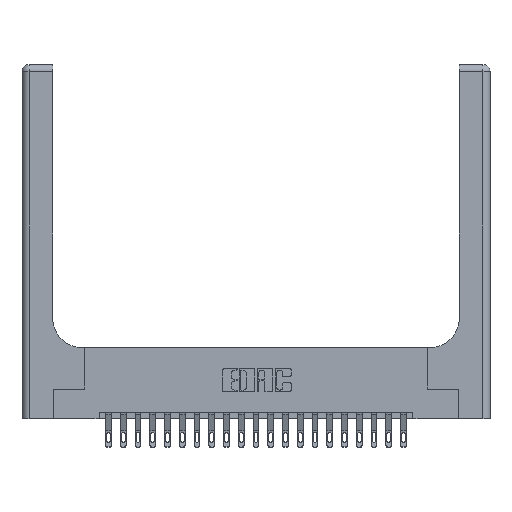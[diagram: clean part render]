
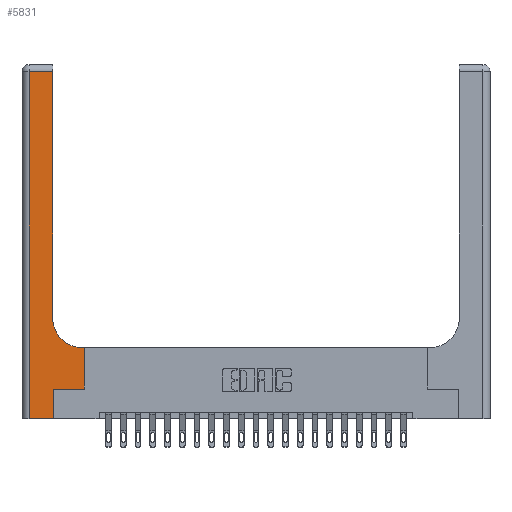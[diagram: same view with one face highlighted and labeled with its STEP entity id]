
A CAD part, top view. The second image highlights one B-rep face of the part: STEP entity #5831.
In plain terms, the highlighted planar face has unit normal (0, 0, 1).
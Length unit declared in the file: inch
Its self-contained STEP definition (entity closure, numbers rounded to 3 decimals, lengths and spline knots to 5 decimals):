
#653 = ORIENTED_EDGE ( 'NONE', *, *, #1979, .T. ) ;
#1203 = EDGE_CURVE ( 'NONE', #4812, #17176, #13345, .T. ) ;
#1388 = CARTESIAN_POINT ( 'NONE',  ( 0.06, 0., 0.37 ) ) ;
#1412 = DIRECTION ( 'NONE',  ( 0., 1., 0. ) ) ;
#1979 = EDGE_CURVE ( 'NONE', #17176, #2848, #15249, .T. ) ;
#2100 = ORIENTED_EDGE ( 'NONE', *, *, #11802, .T. ) ;
#2251 = VECTOR ( 'NONE', #11973, 39.37008 ) ;
#2461 = DIRECTION ( 'NONE',  ( -1., 0., 0. ) ) ;
#2636 = CARTESIAN_POINT ( 'NONE',  ( 0.26, 0.6, 0.37 ) ) ;
#2697 = DIRECTION ( 'NONE',  ( 0., 1., 0. ) ) ;
#2848 = VERTEX_POINT ( 'NONE', #14149 ) ;
#3177 = CARTESIAN_POINT ( 'NONE',  ( 0.51, 0.6, 0.37 ) ) ;
#3280 = ORIENTED_EDGE ( 'NONE', *, *, #10974, .T. ) ;
#3754 = CARTESIAN_POINT ( 'NONE',  ( 0.265, 0., 0.37 ) ) ;
#3916 = CARTESIAN_POINT ( 'NONE',  ( 0., 0., 0.37 ) ) ;
#4311 = ORIENTED_EDGE ( 'NONE', *, *, #11282, .T. ) ;
#4402 = CARTESIAN_POINT ( 'NONE',  ( 0.528, 0.25, 0.37 ) ) ;
#4812 = VERTEX_POINT ( 'NONE', #6133 ) ;
#5831 = ADVANCED_FACE ( 'NONE', ( #19494 ), #12582, .F. ) ;
#6133 = CARTESIAN_POINT ( 'NONE',  ( 0.528, 0.6, 0.37 ) ) ;
#6538 = DIRECTION ( 'NONE',  ( 1., 0., 0. ) ) ;
#6682 = DIRECTION ( 'NONE',  ( 1., 0., 0. ) ) ;
#6958 = VERTEX_POINT ( 'NONE', #17287 ) ;
#7157 = ORIENTED_EDGE ( 'NONE', *, *, #1203, .T. ) ;
#7297 = EDGE_CURVE ( 'NONE', #20458, #9499, #17157, .T. ) ;
#7345 = LINE ( 'NONE', #3916, #10226 ) ;
#7365 = VECTOR ( 'NONE', #1412, 39.37008 ) ;
#7454 = AXIS2_PLACEMENT_3D ( 'NONE', #21672, #19728, #16337 ) ;
#8515 = ORIENTED_EDGE ( 'NONE', *, *, #7297, .T. ) ;
#8756 = VECTOR ( 'NONE', #2697, 39.37008 ) ;
#8896 = CARTESIAN_POINT ( 'NONE',  ( 0.265, 0.25, 0.37 ) ) ;
#9025 = CARTESIAN_POINT ( 'NONE',  ( 0.06, 2.94, 0.37 ) ) ;
#9262 = LINE ( 'NONE', #16222, #17305 ) ;
#9431 = VECTOR ( 'NONE', #6538, 39.37008 ) ;
#9499 = VERTEX_POINT ( 'NONE', #15366 ) ;
#10226 = VECTOR ( 'NONE', #19401, 39.37008 ) ;
#10974 = EDGE_CURVE ( 'NONE', #9499, #4812, #19881, .T. ) ;
#11282 = EDGE_CURVE ( 'NONE', #15295, #21851, #7345, .T. ) ;
#11802 = EDGE_CURVE ( 'NONE', #13769, #15295, #16662, .T. ) ;
#11973 = DIRECTION ( 'NONE',  ( 0., -1., 0. ) ) ;
#12073 = LINE ( 'NONE', #19518, #16566 ) ;
#12582 = PLANE ( 'NONE',  #7454 ) ;
#12653 = EDGE_CURVE ( 'NONE', #21851, #20458, #13720, .T. ) ;
#12925 = DIRECTION ( 'NONE',  ( 0., 1., 0. ) ) ;
#13345 = LINE ( 'NONE', #2636, #22180 ) ;
#13720 = LINE ( 'NONE', #15090, #7365 ) ;
#13769 = VERTEX_POINT ( 'NONE', #9025 ) ;
#13984 = CARTESIAN_POINT ( 'NONE',  ( 0.265, 0.25, 0.37 ) ) ;
#14149 = CARTESIAN_POINT ( 'NONE',  ( 0.26, 0.85, 0.37 ) ) ;
#14594 = ORIENTED_EDGE ( 'NONE', *, *, #15842, .T. ) ;
#14723 = ORIENTED_EDGE ( 'NONE', *, *, #12653, .T. ) ;
#15090 = CARTESIAN_POINT ( 'NONE',  ( 0.265, 0., 0.37 ) ) ;
#15249 = CIRCLE ( 'NONE', #21036, 0.25 ) ;
#15295 = VERTEX_POINT ( 'NONE', #1388 ) ;
#15366 = CARTESIAN_POINT ( 'NONE',  ( 0.528, 0.25, 0.37 ) ) ;
#15541 = ORIENTED_EDGE ( 'NONE', *, *, #16476, .T. ) ;
#15842 = EDGE_CURVE ( 'NONE', #6958, #13769, #12073, .T. ) ;
#16222 = CARTESIAN_POINT ( 'NONE',  ( 0.26, 3., 0.37 ) ) ;
#16337 = DIRECTION ( 'NONE',  ( -1., 0., 0. ) ) ;
#16476 = EDGE_CURVE ( 'NONE', #2848, #6958, #9262, .T. ) ;
#16566 = VECTOR ( 'NONE', #2461, 39.37008 ) ;
#16662 = LINE ( 'NONE', #18469, #2251 ) ;
#17157 = LINE ( 'NONE', #8896, #9431 ) ;
#17176 = VERTEX_POINT ( 'NONE', #3177 ) ;
#17287 = CARTESIAN_POINT ( 'NONE',  ( 0.26, 2.94, 0.37 ) ) ;
#17305 = VECTOR ( 'NONE', #12925, 39.37008 ) ;
#18459 = EDGE_LOOP ( 'NONE', ( #15541, #14594, #2100, #4311, #14723, #8515, #3280, #7157, #653 ) ) ;
#18469 = CARTESIAN_POINT ( 'NONE',  ( 0.06, 3., 0.37 ) ) ;
#18989 = DIRECTION ( 'NONE',  ( 0., 0., -1. ) ) ;
#19401 = DIRECTION ( 'NONE',  ( 1., 0., 0. ) ) ;
#19494 = FACE_OUTER_BOUND ( 'NONE', #18459, .T. ) ;
#19518 = CARTESIAN_POINT ( 'NONE',  ( 0., 2.94, 0.37 ) ) ;
#19728 = DIRECTION ( 'NONE',  ( 0., 0., -1. ) ) ;
#19881 = LINE ( 'NONE', #4402, #8756 ) ;
#20458 = VERTEX_POINT ( 'NONE', #13984 ) ;
#21036 = AXIS2_PLACEMENT_3D ( 'NONE', #22284, #18989, #6682 ) ;
#21672 = CARTESIAN_POINT ( 'NONE',  ( 0., 3., 0.37 ) ) ;
#21851 = VERTEX_POINT ( 'NONE', #3754 ) ;
#22180 = VECTOR ( 'NONE', #22196, 39.37008 ) ;
#22196 = DIRECTION ( 'NONE',  ( -1., 0., 0. ) ) ;
#22284 = CARTESIAN_POINT ( 'NONE',  ( 0.51, 0.85, 0.37 ) ) ;
